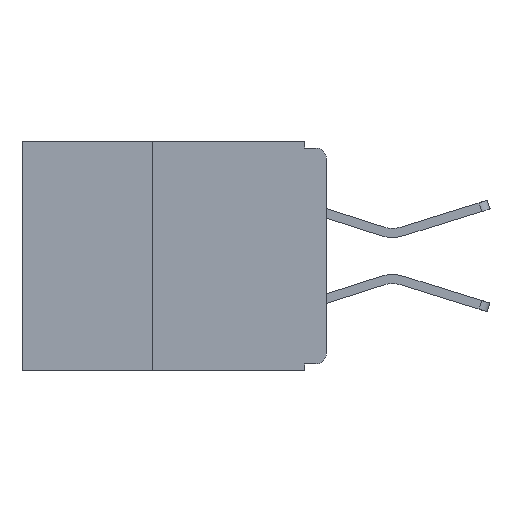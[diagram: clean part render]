
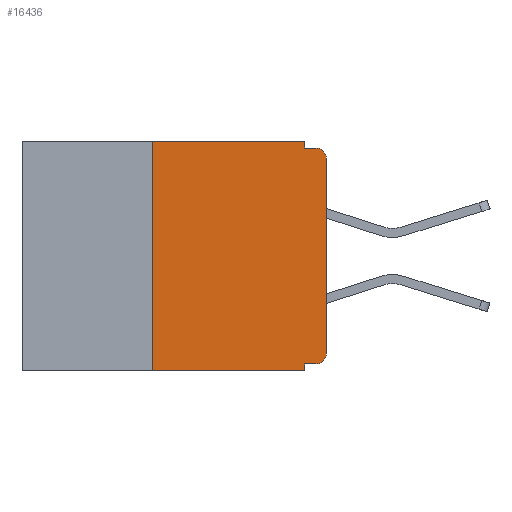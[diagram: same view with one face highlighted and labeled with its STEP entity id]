
A CAD part, left-side view. The second image highlights one B-rep face of the part: STEP entity #16436.
In plain terms, the highlighted planar face has unit normal (-1, 0, 0).
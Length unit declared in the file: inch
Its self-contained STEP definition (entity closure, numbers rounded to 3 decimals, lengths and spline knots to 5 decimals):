
#103 = VECTOR ( 'NONE', #6313, 39.37008 ) ;
#888 = CARTESIAN_POINT ( 'NONE',  ( 0., 0.031, -0.01 ) ) ;
#964 = CARTESIAN_POINT ( 'NONE',  ( 0., 0.015, -0.305 ) ) ;
#1085 = VERTEX_POINT ( 'NONE', #6621 ) ;
#1599 = VECTOR ( 'NONE', #22979, 39.37008 ) ;
#1638 = CARTESIAN_POINT ( 'NONE',  ( 0., 0.437, 0. ) ) ;
#1657 = ORIENTED_EDGE ( 'NONE', *, *, #3995, .F. ) ;
#1963 = ORIENTED_EDGE ( 'NONE', *, *, #20763, .F. ) ;
#2282 = CARTESIAN_POINT ( 'NONE',  ( 0., 0.015, -0.025 ) ) ;
#2356 = ORIENTED_EDGE ( 'NONE', *, *, #9984, .F. ) ;
#2367 = VERTEX_POINT ( 'NONE', #6545 ) ;
#2561 = CARTESIAN_POINT ( 'NONE',  ( 0., 0., -0.025 ) ) ;
#2911 = DIRECTION ( 'NONE',  ( 0., 0., -1. ) ) ;
#3400 = DIRECTION ( 'NONE',  ( 0., 1., 0. ) ) ;
#3572 = CARTESIAN_POINT ( 'NONE',  ( 0., 0.25, 0. ) ) ;
#3995 = EDGE_CURVE ( 'NONE', #2367, #12071, #10072, .T. ) ;
#4173 = VERTEX_POINT ( 'NONE', #18624 ) ;
#4216 = DIRECTION ( 'NONE',  ( 0., 0., -1. ) ) ;
#4635 = CARTESIAN_POINT ( 'NONE',  ( 0., 0., -0.305 ) ) ;
#5004 = VECTOR ( 'NONE', #24184, 39.37008 ) ;
#5303 = ORIENTED_EDGE ( 'NONE', *, *, #20037, .F. ) ;
#5633 = ORIENTED_EDGE ( 'NONE', *, *, #22735, .T. ) ;
#5796 = DIRECTION ( 'NONE',  ( 0., -1., 0. ) ) ;
#6289 = ORIENTED_EDGE ( 'NONE', *, *, #13008, .T. ) ;
#6313 = DIRECTION ( 'NONE',  ( 0., 0., 1. ) ) ;
#6545 = CARTESIAN_POINT ( 'NONE',  ( 0., 0.031, 0. ) ) ;
#6554 = VERTEX_POINT ( 'NONE', #4635 ) ;
#6609 = LINE ( 'NONE', #15437, #11058 ) ;
#6621 = CARTESIAN_POINT ( 'NONE',  ( 0., 0.031, -0.33 ) ) ;
#6706 = LINE ( 'NONE', #22891, #1599 ) ;
#6915 = ORIENTED_EDGE ( 'NONE', *, *, #15313, .T. ) ;
#7012 = LINE ( 'NONE', #8607, #21963 ) ;
#7454 = DIRECTION ( 'NONE',  ( 0., 0., -1. ) ) ;
#7858 = DIRECTION ( 'NONE',  ( 0., 0., -1. ) ) ;
#8405 = VECTOR ( 'NONE', #5796, 39.37008 ) ;
#8607 = CARTESIAN_POINT ( 'NONE',  ( 0., 0., 0. ) ) ;
#8756 = ORIENTED_EDGE ( 'NONE', *, *, #13078, .F. ) ;
#9341 = LINE ( 'NONE', #14744, #19322 ) ;
#9453 = AXIS2_PLACEMENT_3D ( 'NONE', #964, #14273, #2911 ) ;
#9478 = CIRCLE ( 'NONE', #9453, 0.015 ) ;
#9984 = EDGE_CURVE ( 'NONE', #11499, #2367, #6706, .T. ) ;
#10072 = LINE ( 'NONE', #21096, #5004 ) ;
#10533 = VERTEX_POINT ( 'NONE', #16493 ) ;
#11058 = VECTOR ( 'NONE', #7858, 39.37008 ) ;
#11468 = CIRCLE ( 'NONE', #22892, 0.015 ) ;
#11499 = VERTEX_POINT ( 'NONE', #3572 ) ;
#11967 = VECTOR ( 'NONE', #22651, 39.37008 ) ;
#12071 = VERTEX_POINT ( 'NONE', #888 ) ;
#13008 = EDGE_CURVE ( 'NONE', #14370, #10533, #11468, .T. ) ;
#13041 = VERTEX_POINT ( 'NONE', #15658 ) ;
#13078 = EDGE_CURVE ( 'NONE', #4173, #11499, #19688, .T. ) ;
#13429 = ORIENTED_EDGE ( 'NONE', *, *, #14625, .F. ) ;
#13860 = EDGE_CURVE ( 'NONE', #6554, #14370, #7012, .T. ) ;
#14273 = DIRECTION ( 'NONE',  ( -1., 0., 0. ) ) ;
#14370 = VERTEX_POINT ( 'NONE', #2561 ) ;
#14598 = LINE ( 'NONE', #24470, #8405 ) ;
#14625 = EDGE_CURVE ( 'NONE', #24375, #13041, #9341, .T. ) ;
#14744 = CARTESIAN_POINT ( 'NONE',  ( 0., 0., -0.32 ) ) ;
#15313 = EDGE_CURVE ( 'NONE', #4173, #1085, #14598, .T. ) ;
#15437 = CARTESIAN_POINT ( 'NONE',  ( 0., 0.031, -0.33 ) ) ;
#15569 = DIRECTION ( 'NONE',  ( -1., 0., 0. ) ) ;
#15658 = CARTESIAN_POINT ( 'NONE',  ( 0., 0.031, -0.32 ) ) ;
#15998 = CARTESIAN_POINT ( 'NONE',  ( 0., 0.015, -0.32 ) ) ;
#16436 = ADVANCED_FACE ( 'NONE', ( #18642 ), #20495, .F. ) ;
#16493 = CARTESIAN_POINT ( 'NONE',  ( 0., 0.015, -0.01 ) ) ;
#17003 = LINE ( 'NONE', #20826, #11967 ) ;
#17163 = ORIENTED_EDGE ( 'NONE', *, *, #13860, .T. ) ;
#17377 = AXIS2_PLACEMENT_3D ( 'NONE', #1638, #18690, #7454 ) ;
#18624 = CARTESIAN_POINT ( 'NONE',  ( 0., 0.25, -0.33 ) ) ;
#18642 = FACE_OUTER_BOUND ( 'NONE', #21126, .T. ) ;
#18690 = DIRECTION ( 'NONE',  ( 1., 0., 0. ) ) ;
#19322 = VECTOR ( 'NONE', #3400, 39.37008 ) ;
#19688 = LINE ( 'NONE', #21278, #103 ) ;
#20037 = EDGE_CURVE ( 'NONE', #12071, #10533, #17003, .T. ) ;
#20495 = PLANE ( 'NONE',  #17377 ) ;
#20763 = EDGE_CURVE ( 'NONE', #13041, #1085, #6609, .T. ) ;
#20826 = CARTESIAN_POINT ( 'NONE',  ( 0., 0., -0.01 ) ) ;
#21096 = CARTESIAN_POINT ( 'NONE',  ( 0., 0.031, 0. ) ) ;
#21126 = EDGE_LOOP ( 'NONE', ( #17163, #6289, #5303, #1657, #2356, #8756, #6915, #1963, #13429, #5633 ) ) ;
#21278 = CARTESIAN_POINT ( 'NONE',  ( 0., 0.25, -0.33 ) ) ;
#21963 = VECTOR ( 'NONE', #23558, 39.37008 ) ;
#22651 = DIRECTION ( 'NONE',  ( 0., -1., 0. ) ) ;
#22735 = EDGE_CURVE ( 'NONE', #24375, #6554, #9478, .T. ) ;
#22891 = CARTESIAN_POINT ( 'NONE',  ( 0., 0.437, 0. ) ) ;
#22892 = AXIS2_PLACEMENT_3D ( 'NONE', #2282, #15569, #4216 ) ;
#22979 = DIRECTION ( 'NONE',  ( 0., -1., 0. ) ) ;
#23558 = DIRECTION ( 'NONE',  ( 0., 0., 1. ) ) ;
#24184 = DIRECTION ( 'NONE',  ( 0., 0., -1. ) ) ;
#24375 = VERTEX_POINT ( 'NONE', #15998 ) ;
#24470 = CARTESIAN_POINT ( 'NONE',  ( 0., 0.437, -0.33 ) ) ;
